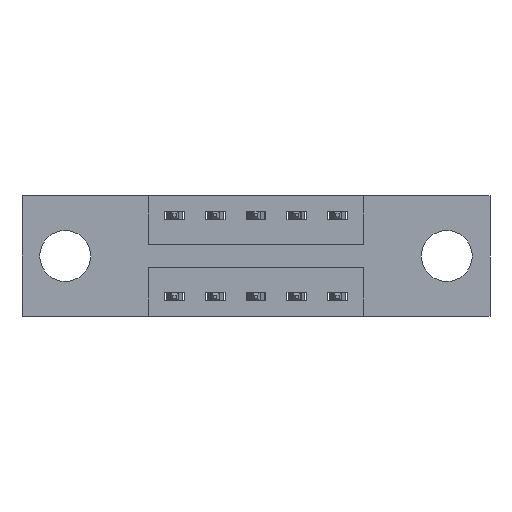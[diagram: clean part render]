
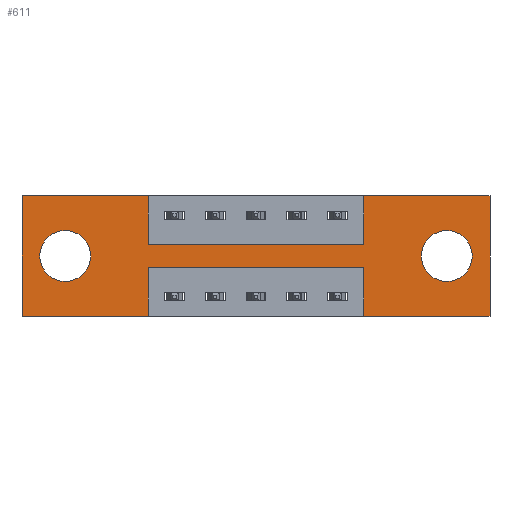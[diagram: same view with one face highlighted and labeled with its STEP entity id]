
A CAD part, front view. The second image highlights one B-rep face of the part: STEP entity #611.
In plain terms, the highlighted planar face has unit normal (0, -1, 0).
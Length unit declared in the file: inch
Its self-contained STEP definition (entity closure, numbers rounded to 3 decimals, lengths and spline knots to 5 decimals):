
#28 = AXIS2_PLACEMENT_3D ( 'NONE', #5881, #1852, #2653 ) ;
#29 = ORIENTED_EDGE ( 'NONE', *, *, #3102, .F. ) ;
#117 = ORIENTED_EDGE ( 'NONE', *, *, #1989, .F. ) ;
#223 = ORIENTED_EDGE ( 'NONE', *, *, #3565, .F. ) ;
#299 = ORIENTED_EDGE ( 'NONE', *, *, #3561, .F. ) ;
#307 = ORIENTED_EDGE ( 'NONE', *, *, #3551, .F. ) ;
#329 = ORIENTED_EDGE ( 'NONE', *, *, #2329, .F. ) ;
#351 = EDGE_CURVE ( 'NONE', #5303, #1226, #5263, .T. ) ;
#360 = DIRECTION ( 'NONE',  ( 0., 0., -1. ) ) ;
#479 = ORIENTED_EDGE ( 'NONE', *, *, #3099, .F. ) ;
#494 = ORIENTED_EDGE ( 'NONE', *, *, #3149, .F. ) ;
#598 = CARTESIAN_POINT ( 'NONE',  ( 0., 0., -0.37 ) ) ;
#611 = ADVANCED_FACE ( 'NONE', ( #4311, #4284, #4327 ), #4365, .T. ) ;
#728 = AXIS2_PLACEMENT_3D ( 'NONE', #4754, #4708, #4747 ) ;
#816 = DIRECTION ( 'NONE',  ( 0., 0., 1. ) ) ;
#853 = DIRECTION ( 'NONE',  ( 0., 1., 0. ) ) ;
#879 = CARTESIAN_POINT ( 'NONE',  ( 0.1325, 0., -0.185 ) ) ;
#1050 = DIRECTION ( 'NONE',  ( 0., 0., -1. ) ) ;
#1055 = CARTESIAN_POINT ( 'NONE',  ( 1.435, 0., -0.37 ) ) ;
#1075 = CARTESIAN_POINT ( 'NONE',  ( 0.3875, 0., -0.22 ) ) ;
#1160 = DIRECTION ( 'NONE',  ( -1., 0., 0. ) ) ;
#1185 = CARTESIAN_POINT ( 'NONE',  ( 0.3875, 0., -0.37 ) ) ;
#1226 = VERTEX_POINT ( 'NONE', #4321 ) ;
#1232 = DIRECTION ( 'NONE',  ( 0., 0., 1. ) ) ;
#1246 = ORIENTED_EDGE ( 'NONE', *, *, #3352, .T. ) ;
#1319 = ORIENTED_EDGE ( 'NONE', *, *, #351, .T. ) ;
#1323 = DIRECTION ( 'NONE',  ( 0., 0., 1. ) ) ;
#1345 = DIRECTION ( 'NONE',  ( 1., 0., 0. ) ) ;
#1361 = CARTESIAN_POINT ( 'NONE',  ( 1.0475, 0., -0.37 ) ) ;
#1380 = CARTESIAN_POINT ( 'NONE',  ( 1.0475, 0., 0. ) ) ;
#1399 = CARTESIAN_POINT ( 'NONE',  ( 0.3875, 0., -0.15 ) ) ;
#1436 = CARTESIAN_POINT ( 'NONE',  ( 0.3875, 0., 0. ) ) ;
#1445 = CARTESIAN_POINT ( 'NONE',  ( 1.0475, 0., -0.22 ) ) ;
#1449 = DIRECTION ( 'NONE',  ( 0., 0., -1. ) ) ;
#1545 = VERTEX_POINT ( 'NONE', #1834 ) ;
#1722 = ORIENTED_EDGE ( 'NONE', *, *, #3682, .T. ) ;
#1834 = CARTESIAN_POINT ( 'NONE',  ( 1.0475, 0., 0. ) ) ;
#1852 = DIRECTION ( 'NONE',  ( 0., 1., 0. ) ) ;
#1989 = EDGE_CURVE ( 'NONE', #1545, #3991, #6898, .T. ) ;
#2025 = CIRCLE ( 'NONE', #728, 0.078 ) ;
#2329 = EDGE_CURVE ( 'NONE', #7147, #6972, #5889, .T. ) ;
#2423 = CARTESIAN_POINT ( 'NONE',  ( 0., 0., 0. ) ) ;
#2471 = CARTESIAN_POINT ( 'NONE',  ( 0.3875, 0., -0.15 ) ) ;
#2653 = DIRECTION ( 'NONE',  ( 0., 0., -1. ) ) ;
#2703 = DIRECTION ( 'NONE',  ( 0., 0., -1. ) ) ;
#2716 = DIRECTION ( 'NONE',  ( 0., 1., 0. ) ) ;
#2720 = CARTESIAN_POINT ( 'NONE',  ( 1.3025, 0., -0.185 ) ) ;
#2755 = DIRECTION ( 'NONE',  ( 1., 0., 0. ) ) ;
#2894 = CARTESIAN_POINT ( 'NONE',  ( 0.3875, 0., -0.37 ) ) ;
#2947 = CIRCLE ( 'NONE', #4292, 0.078 ) ;
#2983 = VECTOR ( 'NONE', #1050, 39.37008 ) ;
#3089 = VECTOR ( 'NONE', #1232, 39.37008 ) ;
#3095 = LINE ( 'NONE', #1361, #3089 ) ;
#3098 = VECTOR ( 'NONE', #1160, 39.37008 ) ;
#3099 = EDGE_CURVE ( 'NONE', #5242, #7147, #4615, .T. ) ;
#3102 = EDGE_CURVE ( 'NONE', #3991, #4952, #4503, .T. ) ;
#3105 = CARTESIAN_POINT ( 'NONE',  ( 0., 0., 0. ) ) ;
#3106 = VECTOR ( 'NONE', #1323, 39.37008 ) ;
#3114 = LINE ( 'NONE', #1075, #3098 ) ;
#3118 = EDGE_CURVE ( 'NONE', #4952, #5887, #4442, .T. ) ;
#3123 = VECTOR ( 'NONE', #1345, 39.37008 ) ;
#3149 = EDGE_CURVE ( 'NONE', #7177, #5242, #4373, .T. ) ;
#3191 = LINE ( 'NONE', #1185, #2983 ) ;
#3196 = VECTOR ( 'NONE', #1449, 39.37008 ) ;
#3201 = LINE ( 'NONE', #1399, #3123 ) ;
#3239 = LINE ( 'NONE', #1436, #3196 ) ;
#3294 = LINE ( 'NONE', #1380, #3106 ) ;
#3352 = EDGE_CURVE ( 'NONE', #1226, #5303, #3762, .T. ) ;
#3551 = EDGE_CURVE ( 'NONE', #6972, #7235, #3239, .T. ) ;
#3561 = EDGE_CURVE ( 'NONE', #7235, #6943, #3201, .T. ) ;
#3565 = EDGE_CURVE ( 'NONE', #6943, #1545, #3294, .T. ) ;
#3576 = EDGE_CURVE ( 'NONE', #5887, #7394, #3095, .T. ) ;
#3657 = EDGE_CURVE ( 'NONE', #7394, #4285, #3114, .T. ) ;
#3661 = EDGE_CURVE ( 'NONE', #4285, #7177, #3191, .T. ) ;
#3682 = EDGE_CURVE ( 'NONE', #7973, #5837, #2947, .T. ) ;
#3762 = CIRCLE ( 'NONE', #4509, 0.078 ) ;
#3814 = CARTESIAN_POINT ( 'NONE',  ( 0.3875, 0., 0. ) ) ;
#3886 = CARTESIAN_POINT ( 'NONE',  ( 1.0475, 0., -0.15 ) ) ;
#3991 = VERTEX_POINT ( 'NONE', #6565 ) ;
#4054 = ORIENTED_EDGE ( 'NONE', *, *, #4413, .T. ) ;
#4136 = ORIENTED_EDGE ( 'NONE', *, *, #3661, .F. ) ;
#4226 = DIRECTION ( 'NONE',  ( -1., 0., 0. ) ) ;
#4251 = CARTESIAN_POINT ( 'NONE',  ( 0., 0., -0.37 ) ) ;
#4284 = FACE_BOUND ( 'NONE', #5964, .T. ) ;
#4285 = VERTEX_POINT ( 'NONE', #5267 ) ;
#4292 = AXIS2_PLACEMENT_3D ( 'NONE', #879, #853, #816 ) ;
#4311 = FACE_BOUND ( 'NONE', #6792, .T. ) ;
#4321 = CARTESIAN_POINT ( 'NONE',  ( 1.3025, 0., -0.107 ) ) ;
#4327 = FACE_OUTER_BOUND ( 'NONE', #7346, .T. ) ;
#4365 = PLANE ( 'NONE',  #4933 ) ;
#4373 = LINE ( 'NONE', #4251, #4469 ) ;
#4413 = EDGE_CURVE ( 'NONE', #5837, #7973, #2025, .T. ) ;
#4417 = VECTOR ( 'NONE', #4429, 39.37008 ) ;
#4429 = DIRECTION ( 'NONE',  ( -1., 0., 0. ) ) ;
#4442 = LINE ( 'NONE', #4494, #4417 ) ;
#4469 = VECTOR ( 'NONE', #4226, 39.37008 ) ;
#4476 = VECTOR ( 'NONE', #4518, 39.37008 ) ;
#4494 = CARTESIAN_POINT ( 'NONE',  ( 0., 0., -0.37 ) ) ;
#4495 = ORIENTED_EDGE ( 'NONE', *, *, #3657, .F. ) ;
#4501 = ORIENTED_EDGE ( 'NONE', *, *, #3576, .F. ) ;
#4503 = LINE ( 'NONE', #4537, #4476 ) ;
#4509 = AXIS2_PLACEMENT_3D ( 'NONE', #2720, #2716, #2703 ) ;
#4515 = VECTOR ( 'NONE', #4643, 39.37008 ) ;
#4518 = DIRECTION ( 'NONE',  ( 0., 0., -1. ) ) ;
#4537 = CARTESIAN_POINT ( 'NONE',  ( 1.435, 0., 0. ) ) ;
#4615 = LINE ( 'NONE', #4645, #4515 ) ;
#4643 = DIRECTION ( 'NONE',  ( 0., 0., 1. ) ) ;
#4645 = CARTESIAN_POINT ( 'NONE',  ( 0., 0., 0. ) ) ;
#4708 = DIRECTION ( 'NONE',  ( 0., 1., 0. ) ) ;
#4747 = DIRECTION ( 'NONE',  ( 0., 0., 1. ) ) ;
#4754 = CARTESIAN_POINT ( 'NONE',  ( 0.1325, 0., -0.185 ) ) ;
#4926 = ORIENTED_EDGE ( 'NONE', *, *, #3118, .F. ) ;
#4933 = AXIS2_PLACEMENT_3D ( 'NONE', #598, #6743, #360 ) ;
#4952 = VERTEX_POINT ( 'NONE', #1055 ) ;
#5242 = VERTEX_POINT ( 'NONE', #7974 ) ;
#5263 = CIRCLE ( 'NONE', #28, 0.078 ) ;
#5267 = CARTESIAN_POINT ( 'NONE',  ( 0.3875, 0., -0.22 ) ) ;
#5303 = VERTEX_POINT ( 'NONE', #7754 ) ;
#5460 = CARTESIAN_POINT ( 'NONE',  ( 0.1325, 0., -0.107 ) ) ;
#5837 = VERTEX_POINT ( 'NONE', #6775 ) ;
#5881 = CARTESIAN_POINT ( 'NONE',  ( 1.3025, 0., -0.185 ) ) ;
#5887 = VERTEX_POINT ( 'NONE', #6850 ) ;
#5889 = LINE ( 'NONE', #6998, #5902 ) ;
#5902 = VECTOR ( 'NONE', #6979, 39.37008 ) ;
#5964 = EDGE_LOOP ( 'NONE', ( #1722, #4054 ) ) ;
#6565 = CARTESIAN_POINT ( 'NONE',  ( 1.435, 0., 0. ) ) ;
#6743 = DIRECTION ( 'NONE',  ( 0., -1., 0. ) ) ;
#6775 = CARTESIAN_POINT ( 'NONE',  ( 0.1325, 0., -0.263 ) ) ;
#6792 = EDGE_LOOP ( 'NONE', ( #1246, #1319 ) ) ;
#6850 = CARTESIAN_POINT ( 'NONE',  ( 1.0475, 0., -0.37 ) ) ;
#6898 = LINE ( 'NONE', #2423, #6901 ) ;
#6901 = VECTOR ( 'NONE', #2755, 39.37008 ) ;
#6943 = VERTEX_POINT ( 'NONE', #3886 ) ;
#6972 = VERTEX_POINT ( 'NONE', #3814 ) ;
#6979 = DIRECTION ( 'NONE',  ( 1., 0., 0. ) ) ;
#6998 = CARTESIAN_POINT ( 'NONE',  ( 0., 0., 0. ) ) ;
#7147 = VERTEX_POINT ( 'NONE', #3105 ) ;
#7177 = VERTEX_POINT ( 'NONE', #2894 ) ;
#7235 = VERTEX_POINT ( 'NONE', #2471 ) ;
#7346 = EDGE_LOOP ( 'NONE', ( #4136, #4495, #4501, #4926, #29, #117, #223, #299, #307, #329, #479, #494 ) ) ;
#7394 = VERTEX_POINT ( 'NONE', #1445 ) ;
#7754 = CARTESIAN_POINT ( 'NONE',  ( 1.3025, 0., -0.263 ) ) ;
#7973 = VERTEX_POINT ( 'NONE', #5460 ) ;
#7974 = CARTESIAN_POINT ( 'NONE',  ( 0., 0., -0.37 ) ) ;
